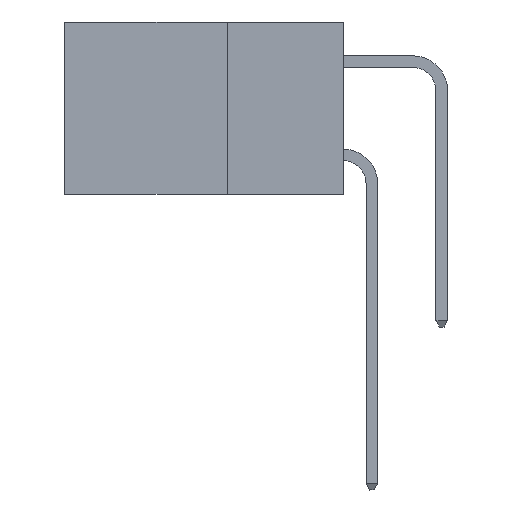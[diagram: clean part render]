
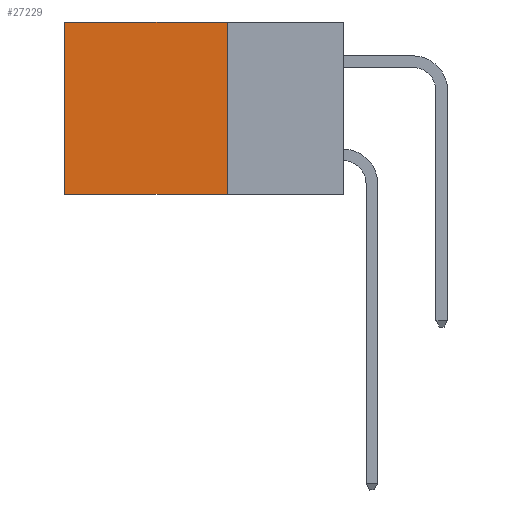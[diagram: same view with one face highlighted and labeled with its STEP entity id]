
A CAD part, left-side view. The second image highlights one B-rep face of the part: STEP entity #27229.
In plain terms, the highlighted planar face has unit normal (-1, 0, 0).
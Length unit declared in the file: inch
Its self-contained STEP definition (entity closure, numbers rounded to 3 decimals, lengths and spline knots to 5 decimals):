
#870 = VERTEX_POINT ( 'NONE', #18361 ) ;
#2749 = LINE ( 'NONE', #3368, #8826 ) ;
#2954 = EDGE_CURVE ( 'NONE', #28281, #13232, #7865, .T. ) ;
#3269 = ORIENTED_EDGE ( 'NONE', *, *, #8132, .F. ) ;
#3368 = CARTESIAN_POINT ( 'NONE',  ( 0.2615, 0.6, -0.37 ) ) ;
#4184 = AXIS2_PLACEMENT_3D ( 'NONE', #4390, #29314, #15885 ) ;
#4390 = CARTESIAN_POINT ( 'NONE',  ( 0.2615, 0.25, -0.37 ) ) ;
#4978 = CARTESIAN_POINT ( 'NONE',  ( 0.2615, 0.6, 0. ) ) ;
#6304 = ORIENTED_EDGE ( 'NONE', *, *, #17642, .T. ) ;
#7865 = LINE ( 'NONE', #13055, #26584 ) ;
#8132 = EDGE_CURVE ( 'NONE', #28493, #870, #13490, .T. ) ;
#8826 = VECTOR ( 'NONE', #19330, 39.37008 ) ;
#11853 = CARTESIAN_POINT ( 'NONE',  ( 0.2615, 0.25, -0.37 ) ) ;
#13055 = CARTESIAN_POINT ( 'NONE',  ( 0.2615, 0.25, 0. ) ) ;
#13127 = DIRECTION ( 'NONE',  ( 0., 1., 0. ) ) ;
#13232 = VERTEX_POINT ( 'NONE', #4978 ) ;
#13490 = LINE ( 'NONE', #14687, #24822 ) ;
#13541 = PLANE ( 'NONE',  #4184 ) ;
#14144 = DIRECTION ( 'NONE',  ( 0., 0., -1. ) ) ;
#14687 = CARTESIAN_POINT ( 'NONE',  ( 0.2615, 0.25, -0.37 ) ) ;
#15132 = VECTOR ( 'NONE', #14144, 39.37008 ) ;
#15783 = CARTESIAN_POINT ( 'NONE',  ( 0.2615, 0.25, 0. ) ) ;
#15885 = DIRECTION ( 'NONE',  ( 0., 0., -1. ) ) ;
#17642 = EDGE_CURVE ( 'NONE', #13232, #870, #2749, .T. ) ;
#18361 = CARTESIAN_POINT ( 'NONE',  ( 0.2615, 0.6, -0.37 ) ) ;
#19330 = DIRECTION ( 'NONE',  ( 0., 0., -1. ) ) ;
#21849 = ORIENTED_EDGE ( 'NONE', *, *, #27407, .F. ) ;
#21870 = LINE ( 'NONE', #11853, #15132 ) ;
#23140 = ORIENTED_EDGE ( 'NONE', *, *, #2954, .T. ) ;
#23169 = EDGE_LOOP ( 'NONE', ( #6304, #3269, #21849, #23140 ) ) ;
#23792 = DIRECTION ( 'NONE',  ( 0., 1., 0. ) ) ;
#24822 = VECTOR ( 'NONE', #23792, 39.37008 ) ;
#26054 = FACE_OUTER_BOUND ( 'NONE', #23169, .T. ) ;
#26584 = VECTOR ( 'NONE', #13127, 39.37008 ) ;
#27229 = ADVANCED_FACE ( 'NONE', ( #26054 ), #13541, .F. ) ;
#27407 = EDGE_CURVE ( 'NONE', #28281, #28493, #21870, .T. ) ;
#27641 = CARTESIAN_POINT ( 'NONE',  ( 0.2615, 0.25, -0.37 ) ) ;
#28281 = VERTEX_POINT ( 'NONE', #15783 ) ;
#28493 = VERTEX_POINT ( 'NONE', #27641 ) ;
#29314 = DIRECTION ( 'NONE',  ( 1., 0., 0. ) ) ;
